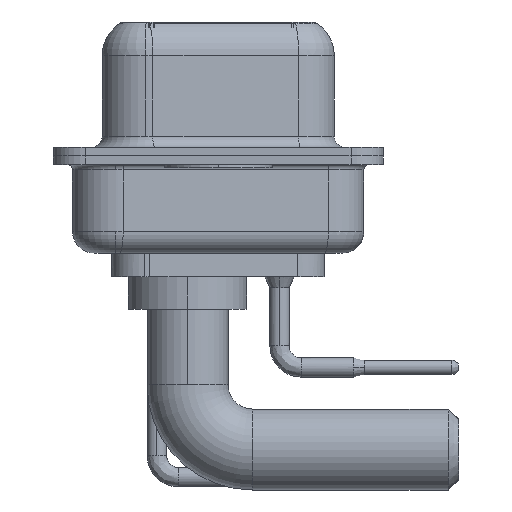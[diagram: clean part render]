
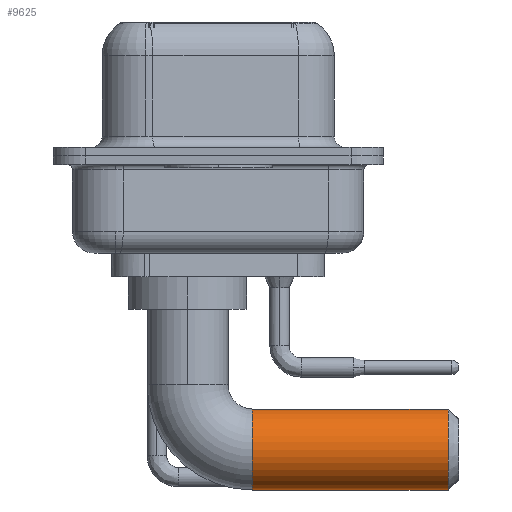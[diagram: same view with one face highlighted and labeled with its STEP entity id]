
A CAD part, left-side view. The second image highlights one B-rep face of the part: STEP entity #9625.
In plain terms, the highlighted cylindrical face has radius 1.875 mm (diameter 3.75 mm), a partial arc.
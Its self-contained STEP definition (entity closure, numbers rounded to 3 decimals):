
#1088 = DIRECTION ( 'NONE',  ( 0., 0., -1. ) ) ;
#1149 = VECTOR ( 'NONE', #22438, 1000. ) ;
#1658 = CARTESIAN_POINT ( 'NONE',  ( 0., -3., -8.375 ) ) ;
#2590 = CARTESIAN_POINT ( 'NONE',  ( 0., -3., -8.375 ) ) ;
#3489 = DIRECTION ( 'NONE',  ( 0., 1., 0. ) ) ;
#3893 = DIRECTION ( 'NONE',  ( 0., -1., 0. ) ) ;
#3992 = AXIS2_PLACEMENT_3D ( 'NONE', #11977, #22689, #1088 ) ;
#4115 = EDGE_CURVE ( 'NONE', #17837, #25413, #5083, .T. ) ;
#4720 = CIRCLE ( 'NONE', #11403, 1.875 ) ;
#5083 = CIRCLE ( 'NONE', #17996, 1.875 ) ;
#7267 = CARTESIAN_POINT ( 'NONE',  ( 0., -12.07, -6.5 ) ) ;
#9485 = DIRECTION ( 'NONE',  ( 0., 0., -1. ) ) ;
#9625 = ADVANCED_FACE ( 'NONE', ( #24505 ), #17838, .T. ) ;
#11403 = AXIS2_PLACEMENT_3D ( 'NONE', #19216, #3893, #20903 ) ;
#11923 = CARTESIAN_POINT ( 'NONE',  ( 0., -12.07, -8.375 ) ) ;
#11977 = CARTESIAN_POINT ( 'NONE',  ( 0., -3., -6.5 ) ) ;
#13800 = CARTESIAN_POINT ( 'NONE',  ( 0., -3., -4.625 ) ) ;
#13824 = ORIENTED_EDGE ( 'NONE', *, *, #25577, .T. ) ;
#15319 = DIRECTION ( 'NONE',  ( 0., -1., 0. ) ) ;
#17837 = VERTEX_POINT ( 'NONE', #11923 ) ;
#17838 = CYLINDRICAL_SURFACE ( 'NONE', #3992, 1.875 ) ;
#17996 = AXIS2_PLACEMENT_3D ( 'NONE', #7267, #3489, #9485 ) ;
#18481 = ORIENTED_EDGE ( 'NONE', *, *, #4115, .T. ) ;
#19216 = CARTESIAN_POINT ( 'NONE',  ( 0., -3., -6.5 ) ) ;
#20350 = VERTEX_POINT ( 'NONE', #13800 ) ;
#20497 = LINE ( 'NONE', #1658, #1149 ) ;
#20903 = DIRECTION ( 'NONE',  ( -1., 0., 0. ) ) ;
#21425 = ORIENTED_EDGE ( 'NONE', *, *, #25403, .T. ) ;
#22302 = CARTESIAN_POINT ( 'NONE',  ( 0., -12.07, -4.625 ) ) ;
#22317 = EDGE_LOOP ( 'NONE', ( #22424, #13824, #21425, #18481 ) ) ;
#22424 = ORIENTED_EDGE ( 'NONE', *, *, #25838, .F. ) ;
#22438 = DIRECTION ( 'NONE',  ( 0., -1., 0. ) ) ;
#22689 = DIRECTION ( 'NONE',  ( 0., -1., 0. ) ) ;
#24226 = CARTESIAN_POINT ( 'NONE',  ( 0., -3., -4.625 ) ) ;
#24505 = FACE_OUTER_BOUND ( 'NONE', #22317, .T. ) ;
#24776 = VECTOR ( 'NONE', #15319, 1000. ) ;
#25403 = EDGE_CURVE ( 'NONE', #26195, #17837, #20497, .T. ) ;
#25413 = VERTEX_POINT ( 'NONE', #22302 ) ;
#25577 = EDGE_CURVE ( 'NONE', #20350, #26195, #4720, .T. ) ;
#25838 = EDGE_CURVE ( 'NONE', #20350, #25413, #25887, .T. ) ;
#25887 = LINE ( 'NONE', #24226, #24776 ) ;
#26195 = VERTEX_POINT ( 'NONE', #2590 ) ;
